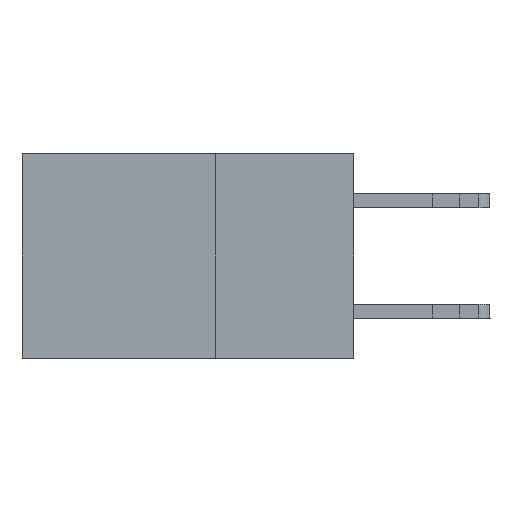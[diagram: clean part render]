
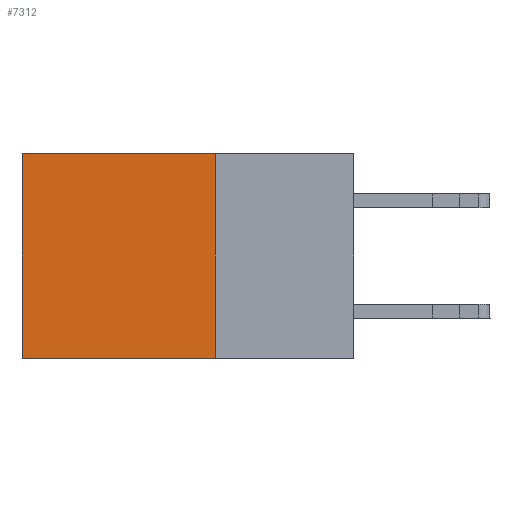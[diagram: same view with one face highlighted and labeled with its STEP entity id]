
A CAD part, left-side view. The second image highlights one B-rep face of the part: STEP entity #7312.
In plain terms, the highlighted planar face has unit normal (-1, 0, 0).
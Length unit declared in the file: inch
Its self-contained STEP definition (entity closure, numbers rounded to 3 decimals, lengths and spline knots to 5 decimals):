
#237 = CARTESIAN_POINT ( 'NONE',  ( 0.2875, 0.25, 0. ) ) ;
#339 = VECTOR ( 'NONE', #7165, 39.37008 ) ;
#745 = ORIENTED_EDGE ( 'NONE', *, *, #3857, .F. ) ;
#1259 = VERTEX_POINT ( 'NONE', #9639 ) ;
#2409 = AXIS2_PLACEMENT_3D ( 'NONE', #7984, #9666, #20996 ) ;
#3082 = LINE ( 'NONE', #13320, #19990 ) ;
#3194 = ORIENTED_EDGE ( 'NONE', *, *, #13186, .F. ) ;
#3240 = ORIENTED_EDGE ( 'NONE', *, *, #6080, .T. ) ;
#3857 = EDGE_CURVE ( 'NONE', #20309, #1259, #3082, .T. ) ;
#4613 = EDGE_CURVE ( 'NONE', #20309, #12978, #6119, .T. ) ;
#5992 = FACE_OUTER_BOUND ( 'NONE', #15381, .T. ) ;
#6080 = EDGE_CURVE ( 'NONE', #12978, #14385, #7883, .T. ) ;
#6119 = LINE ( 'NONE', #237, #14492 ) ;
#7165 = DIRECTION ( 'NONE',  ( 0., 1., 0. ) ) ;
#7312 = ADVANCED_FACE ( 'NONE', ( #5992 ), #19396, .F. ) ;
#7883 = LINE ( 'NONE', #11144, #15672 ) ;
#7984 = CARTESIAN_POINT ( 'NONE',  ( 0.2875, 0.25, 0. ) ) ;
#8325 = DIRECTION ( 'NONE',  ( 0., 0., -1. ) ) ;
#9639 = CARTESIAN_POINT ( 'NONE',  ( 0.2875, 0.25, -0.37 ) ) ;
#9666 = DIRECTION ( 'NONE',  ( 1., 0., 0. ) ) ;
#11144 = CARTESIAN_POINT ( 'NONE',  ( 0.2875, 0.6, 0. ) ) ;
#11228 = CARTESIAN_POINT ( 'NONE',  ( 0.2875, 0.6, -0.37 ) ) ;
#11921 = ORIENTED_EDGE ( 'NONE', *, *, #4613, .T. ) ;
#12978 = VERTEX_POINT ( 'NONE', #16577 ) ;
#13186 = EDGE_CURVE ( 'NONE', #1259, #14385, #17732, .T. ) ;
#13320 = CARTESIAN_POINT ( 'NONE',  ( 0.2875, 0.25, 0. ) ) ;
#13515 = DIRECTION ( 'NONE',  ( 0., 1., 0. ) ) ;
#14385 = VERTEX_POINT ( 'NONE', #11228 ) ;
#14492 = VECTOR ( 'NONE', #13515, 39.37008 ) ;
#15381 = EDGE_LOOP ( 'NONE', ( #3240, #3194, #745, #11921 ) ) ;
#15460 = CARTESIAN_POINT ( 'NONE',  ( 0.2875, 0.25, -0.37 ) ) ;
#15672 = VECTOR ( 'NONE', #16192, 39.37008 ) ;
#16192 = DIRECTION ( 'NONE',  ( 0., 0., -1. ) ) ;
#16577 = CARTESIAN_POINT ( 'NONE',  ( 0.2875, 0.6, 0. ) ) ;
#17732 = LINE ( 'NONE', #15460, #339 ) ;
#17869 = CARTESIAN_POINT ( 'NONE',  ( 0.2875, 0.25, 0. ) ) ;
#19396 = PLANE ( 'NONE',  #2409 ) ;
#19990 = VECTOR ( 'NONE', #8325, 39.37008 ) ;
#20309 = VERTEX_POINT ( 'NONE', #17869 ) ;
#20996 = DIRECTION ( 'NONE',  ( 0., 0., -1. ) ) ;
